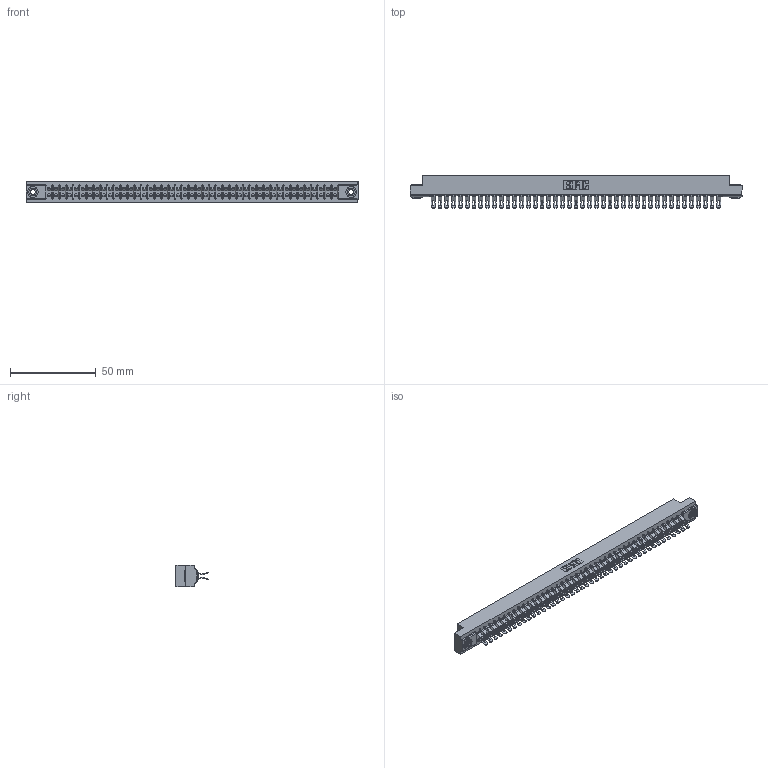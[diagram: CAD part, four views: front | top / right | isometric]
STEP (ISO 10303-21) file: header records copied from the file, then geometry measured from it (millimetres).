
FILE_DESCRIPTION (( 'STEP AP203' ), '1' );
FILE_NAME ('357-086-455-203.STEP', '2020-10-04T06:10:23', ( '' ), ( '' ), 'SwSTEP 2.0', 'SolidWorks 2020', '' );
FILE_SCHEMA (( 'CONFIG_CONTROL_DESIGN' ));
Length unit declared in the file: inch
Products named in the file (4): 307-290-001_555; 357-086-455-203; 345-250-002_345-250-002-102; 307 Part_.156 Dia Mounting Holes
Assembly tree (89 placements, depth 2):
  357-086-455-203
    307 Part_.156 Dia Mounting Holes
    307-290-001_555  x86
    345-250-002_345-250-002-102  x2
Bounding box: 193.4 x 18.75 x 12.7 mm (x, y, z)
Volume: 20830 mm3; surface area: 27179.5 mm2
Topology: 89 solids, 89 shells, 5460 faces, 16001 edges, 10430 vertices
Faces by surface type: plane 3018, cylinder 2346, sphere 88, cone 8
Entity records: 39718 total; most frequent: CARTESIAN_POINT 6484, ORIENTED_EDGE 6420, DIRECTION 6372, EDGE_CURVE 3210, VECTOR 2444, LINE 2444, VERTEX_POINT 2076, AXIS2_PLACEMENT_3D 1964
